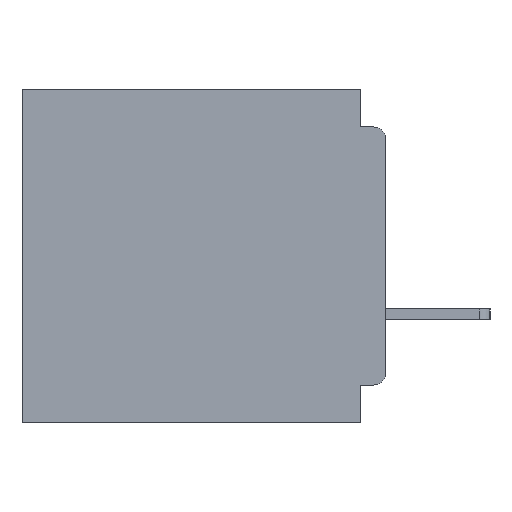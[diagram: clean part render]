
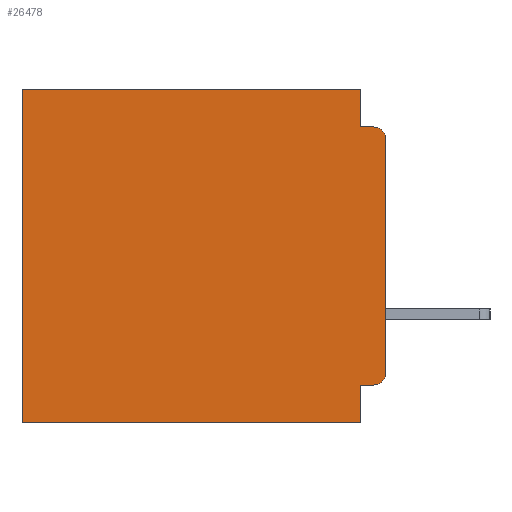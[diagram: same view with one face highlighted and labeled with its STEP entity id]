
A CAD part, left-side view. The second image highlights one B-rep face of the part: STEP entity #26478.
In plain terms, the highlighted planar face has unit normal (-1, 0, 0).
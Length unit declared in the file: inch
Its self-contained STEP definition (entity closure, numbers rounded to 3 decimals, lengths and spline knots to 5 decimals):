
#473 = DIRECTION ( 'NONE',  ( 0., 1., 0. ) ) ;
#1046 = EDGE_CURVE ( 'NONE', #17081, #8028, #32040, .T. ) ;
#1524 = CARTESIAN_POINT ( 'NONE',  ( 0.3, 0., 0. ) ) ;
#1554 = CARTESIAN_POINT ( 'NONE',  ( 0.3, 0.437, -0.4 ) ) ;
#2141 = VERTEX_POINT ( 'NONE', #29301 ) ;
#2663 = ORIENTED_EDGE ( 'NONE', *, *, #7861, .F. ) ;
#2808 = VECTOR ( 'NONE', #12731, 39.37008 ) ;
#3362 = AXIS2_PLACEMENT_3D ( 'NONE', #25255, #7401, #28256 ) ;
#3903 = LINE ( 'NONE', #1524, #18871 ) ;
#4240 = DIRECTION ( 'NONE',  ( -1., 0., 0. ) ) ;
#4425 = CARTESIAN_POINT ( 'NONE',  ( 0.3, 0.015, -0.355 ) ) ;
#5051 = DIRECTION ( 'NONE',  ( 0., 0., -1. ) ) ;
#5300 = VECTOR ( 'NONE', #9158, 39.37008 ) ;
#5412 = CARTESIAN_POINT ( 'NONE',  ( 0.3, 0.031, 0. ) ) ;
#5788 = EDGE_CURVE ( 'NONE', #34559, #6429, #9703, .T. ) ;
#6429 = VERTEX_POINT ( 'NONE', #8516 ) ;
#7200 = EDGE_CURVE ( 'NONE', #6429, #30734, #15654, .T. ) ;
#7348 = EDGE_CURVE ( 'NONE', #12801, #30734, #10050, .T. ) ;
#7401 = DIRECTION ( 'NONE',  ( -1., 0., 0. ) ) ;
#7861 = EDGE_CURVE ( 'NONE', #2141, #21526, #23032, .T. ) ;
#8028 = VERTEX_POINT ( 'NONE', #1554 ) ;
#8516 = CARTESIAN_POINT ( 'NONE',  ( 0.3, 0.031, -0.045 ) ) ;
#9158 = DIRECTION ( 'NONE',  ( 0., 1., 0. ) ) ;
#9272 = EDGE_CURVE ( 'NONE', #37551, #27622, #16937, .T. ) ;
#9703 = LINE ( 'NONE', #5412, #17654 ) ;
#9725 = CARTESIAN_POINT ( 'NONE',  ( 0.3, 0.031, -0.4 ) ) ;
#9766 = PLANE ( 'NONE',  #21399 ) ;
#10050 = CIRCLE ( 'NONE', #3362, 0.015 ) ;
#10276 = CARTESIAN_POINT ( 'NONE',  ( 0.3, 0.437, 0. ) ) ;
#10597 = DIRECTION ( 'NONE',  ( 0., 1., 0. ) ) ;
#10785 = LINE ( 'NONE', #33641, #2808 ) ;
#12590 = DIRECTION ( 'NONE',  ( 0., -1., 0. ) ) ;
#12675 = DIRECTION ( 'NONE',  ( 0., 0., -1. ) ) ;
#12729 = DIRECTION ( 'NONE',  ( 1., 0., 0. ) ) ;
#12731 = DIRECTION ( 'NONE',  ( 0., 0., -1. ) ) ;
#12801 = VERTEX_POINT ( 'NONE', #18201 ) ;
#13243 = LINE ( 'NONE', #18044, #5300 ) ;
#13436 = EDGE_CURVE ( 'NONE', #37551, #2141, #13243, .T. ) ;
#13789 = ORIENTED_EDGE ( 'NONE', *, *, #28868, .F. ) ;
#13876 = CARTESIAN_POINT ( 'NONE',  ( 0.3, 0.437, -0.4 ) ) ;
#14254 = ORIENTED_EDGE ( 'NONE', *, *, #7348, .T. ) ;
#14930 = CARTESIAN_POINT ( 'NONE',  ( 0.3, 0.031, 0. ) ) ;
#15232 = VECTOR ( 'NONE', #5051, 39.37008 ) ;
#15623 = ORIENTED_EDGE ( 'NONE', *, *, #7200, .F. ) ;
#15654 = LINE ( 'NONE', #21606, #29622 ) ;
#15811 = CARTESIAN_POINT ( 'NONE',  ( 0.3, 0., -0.34 ) ) ;
#15918 = ORIENTED_EDGE ( 'NONE', *, *, #5788, .F. ) ;
#16858 = ORIENTED_EDGE ( 'NONE', *, *, #30111, .T. ) ;
#16903 = ORIENTED_EDGE ( 'NONE', *, *, #1046, .T. ) ;
#16937 = CIRCLE ( 'NONE', #26915, 0.015 ) ;
#17081 = VERTEX_POINT ( 'NONE', #10276 ) ;
#17654 = VECTOR ( 'NONE', #20281, 39.37008 ) ;
#18044 = CARTESIAN_POINT ( 'NONE',  ( 0.3, 0., -0.355 ) ) ;
#18201 = CARTESIAN_POINT ( 'NONE',  ( 0.3, 0., -0.06 ) ) ;
#18684 = EDGE_LOOP ( 'NONE', ( #13789, #14254, #15623, #15918, #16858, #16903, #27167, #2663, #32741, #19390 ) ) ;
#18850 = FACE_OUTER_BOUND ( 'NONE', #18684, .T. ) ;
#18871 = VECTOR ( 'NONE', #10597, 39.37008 ) ;
#19390 = ORIENTED_EDGE ( 'NONE', *, *, #9272, .T. ) ;
#19402 = CARTESIAN_POINT ( 'NONE',  ( 0.3, 0.015, -0.045 ) ) ;
#19681 = EDGE_CURVE ( 'NONE', #21526, #8028, #32271, .T. ) ;
#20281 = DIRECTION ( 'NONE',  ( 0., 0., -1. ) ) ;
#21399 = AXIS2_PLACEMENT_3D ( 'NONE', #36507, #12729, #33639 ) ;
#21526 = VERTEX_POINT ( 'NONE', #37652 ) ;
#21606 = CARTESIAN_POINT ( 'NONE',  ( 0.3, 0., -0.045 ) ) ;
#22136 = CARTESIAN_POINT ( 'NONE',  ( 0.3, 0.015, -0.34 ) ) ;
#23032 = LINE ( 'NONE', #9725, #38016 ) ;
#23361 = VECTOR ( 'NONE', #473, 39.37008 ) ;
#24401 = CARTESIAN_POINT ( 'NONE',  ( 0.3, 0., -0.4 ) ) ;
#25138 = DIRECTION ( 'NONE',  ( 0., 0., -1. ) ) ;
#25255 = CARTESIAN_POINT ( 'NONE',  ( 0.3, 0.015, -0.06 ) ) ;
#26478 = ADVANCED_FACE ( 'NONE', ( #18850 ), #9766, .F. ) ;
#26915 = AXIS2_PLACEMENT_3D ( 'NONE', #22136, #4240, #25138 ) ;
#27167 = ORIENTED_EDGE ( 'NONE', *, *, #19681, .F. ) ;
#27622 = VERTEX_POINT ( 'NONE', #15811 ) ;
#28256 = DIRECTION ( 'NONE',  ( 0., 0., -1. ) ) ;
#28868 = EDGE_CURVE ( 'NONE', #12801, #27622, #10785, .T. ) ;
#29301 = CARTESIAN_POINT ( 'NONE',  ( 0.3, 0.031, -0.355 ) ) ;
#29622 = VECTOR ( 'NONE', #12590, 39.37008 ) ;
#30111 = EDGE_CURVE ( 'NONE', #34559, #17081, #3903, .T. ) ;
#30734 = VERTEX_POINT ( 'NONE', #19402 ) ;
#32040 = LINE ( 'NONE', #13876, #15232 ) ;
#32271 = LINE ( 'NONE', #24401, #23361 ) ;
#32741 = ORIENTED_EDGE ( 'NONE', *, *, #13436, .F. ) ;
#33639 = DIRECTION ( 'NONE',  ( 0., 0., -1. ) ) ;
#33641 = CARTESIAN_POINT ( 'NONE',  ( 0.3, 0., -0.4 ) ) ;
#34559 = VERTEX_POINT ( 'NONE', #14930 ) ;
#36507 = CARTESIAN_POINT ( 'NONE',  ( 0.3, 0., -0.4 ) ) ;
#37551 = VERTEX_POINT ( 'NONE', #4425 ) ;
#37652 = CARTESIAN_POINT ( 'NONE',  ( 0.3, 0.031, -0.4 ) ) ;
#38016 = VECTOR ( 'NONE', #12675, 39.37008 ) ;
